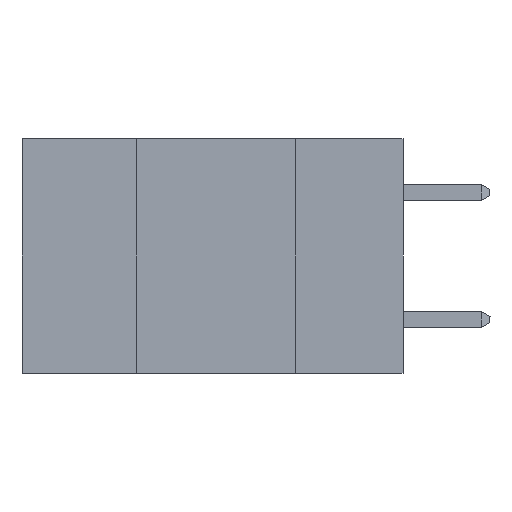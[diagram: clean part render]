
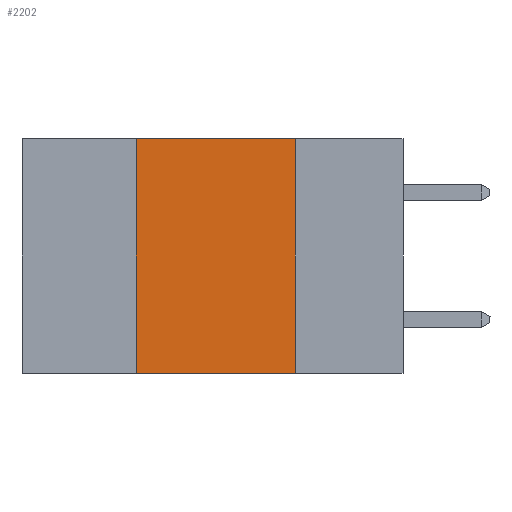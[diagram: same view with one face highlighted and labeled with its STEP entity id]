
A CAD part, left-side view. The second image highlights one B-rep face of the part: STEP entity #2202.
In plain terms, the highlighted planar face has unit normal (-1, 0, 0).
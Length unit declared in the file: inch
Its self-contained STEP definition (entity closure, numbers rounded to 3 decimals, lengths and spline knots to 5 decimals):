
#228 = ORIENTED_EDGE ( 'NONE', *, *, #32894, .F. ) ;
#1958 = DIRECTION ( 'NONE',  ( 0., 0., -1. ) ) ;
#2202 = ADVANCED_FACE ( 'NONE', ( #18952 ), #28239, .F. ) ;
#2585 = LINE ( 'NONE', #31032, #7163 ) ;
#6413 = LINE ( 'NONE', #11754, #40115 ) ;
#7163 = VECTOR ( 'NONE', #24289, 39.37008 ) ;
#11672 = DIRECTION ( 'NONE',  ( 0., -1., 0. ) ) ;
#11754 = CARTESIAN_POINT ( 'NONE',  ( 0., 0.6, 0. ) ) ;
#12437 = EDGE_CURVE ( 'NONE', #35231, #29812, #6413, .T. ) ;
#14249 = VECTOR ( 'NONE', #11672, 39.37008 ) ;
#14886 = CARTESIAN_POINT ( 'NONE',  ( 0., 0.42, 0. ) ) ;
#16832 = DIRECTION ( 'NONE',  ( 0., 0., 1. ) ) ;
#17578 = VERTEX_POINT ( 'NONE', #26827 ) ;
#18952 = FACE_OUTER_BOUND ( 'NONE', #29609, .T. ) ;
#21983 = EDGE_CURVE ( 'NONE', #17578, #32510, #31669, .T. ) ;
#23149 = CARTESIAN_POINT ( 'NONE',  ( 0., 0.42, 0. ) ) ;
#23471 = ORIENTED_EDGE ( 'NONE', *, *, #21983, .T. ) ;
#24289 = DIRECTION ( 'NONE',  ( 0., 0., -1. ) ) ;
#25359 = CARTESIAN_POINT ( 'NONE',  ( 0., 0.6, 0. ) ) ;
#26827 = CARTESIAN_POINT ( 'NONE',  ( 0., 0.42, -0.37 ) ) ;
#27069 = EDGE_CURVE ( 'NONE', #17578, #35231, #35692, .T. ) ;
#28239 = PLANE ( 'NONE',  #33970 ) ;
#28338 = VECTOR ( 'NONE', #16832, 39.37008 ) ;
#29609 = EDGE_LOOP ( 'NONE', ( #228, #31855, #33363, #23471 ) ) ;
#29812 = VERTEX_POINT ( 'NONE', #35018 ) ;
#31032 = CARTESIAN_POINT ( 'NONE',  ( 0., 0.17, 0. ) ) ;
#31669 = LINE ( 'NONE', #31700, #14249 ) ;
#31700 = CARTESIAN_POINT ( 'NONE',  ( 0., 0.6, -0.37 ) ) ;
#31855 = ORIENTED_EDGE ( 'NONE', *, *, #12437, .F. ) ;
#32510 = VERTEX_POINT ( 'NONE', #36169 ) ;
#32894 = EDGE_CURVE ( 'NONE', #29812, #32510, #2585, .T. ) ;
#33363 = ORIENTED_EDGE ( 'NONE', *, *, #27069, .F. ) ;
#33970 = AXIS2_PLACEMENT_3D ( 'NONE', #25359, #34638, #1958 ) ;
#34638 = DIRECTION ( 'NONE',  ( 1., 0., 0. ) ) ;
#35018 = CARTESIAN_POINT ( 'NONE',  ( 0., 0.17, 0. ) ) ;
#35231 = VERTEX_POINT ( 'NONE', #14886 ) ;
#35692 = LINE ( 'NONE', #23149, #28338 ) ;
#36169 = CARTESIAN_POINT ( 'NONE',  ( 0., 0.17, -0.37 ) ) ;
#37869 = DIRECTION ( 'NONE',  ( 0., -1., 0. ) ) ;
#40115 = VECTOR ( 'NONE', #37869, 39.37008 ) ;
